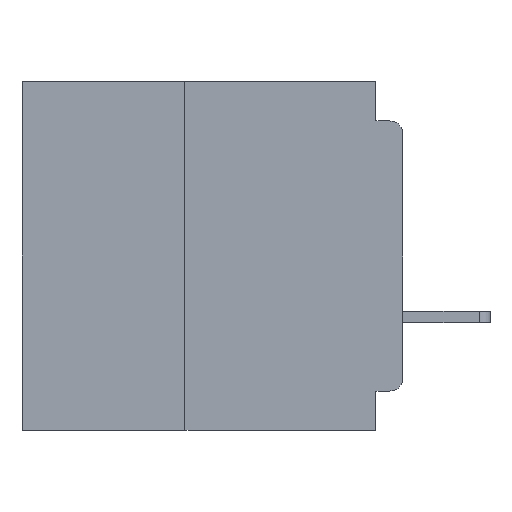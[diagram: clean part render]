
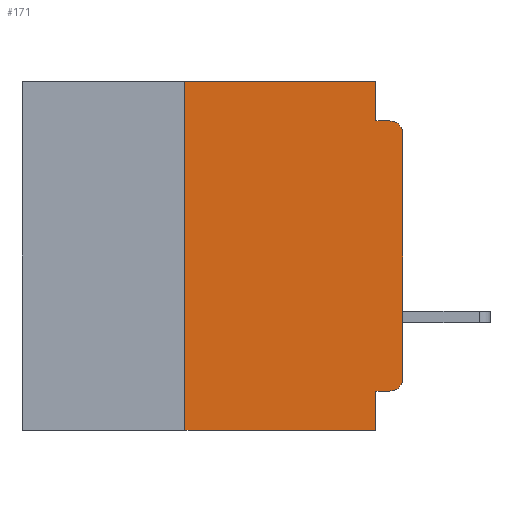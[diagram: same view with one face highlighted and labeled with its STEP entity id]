
A CAD part, left-side view. The second image highlights one B-rep face of the part: STEP entity #171.
In plain terms, the highlighted planar face has unit normal (-1, 0, 0).
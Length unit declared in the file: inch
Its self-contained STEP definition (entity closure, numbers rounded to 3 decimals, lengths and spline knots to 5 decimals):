
#171 = ADVANCED_FACE ( 'NONE', ( #26048 ), #30924, .F. ) ;
#3354 = CARTESIAN_POINT ( 'NONE',  ( 0., 0.031, -0.045 ) ) ;
#3966 = VECTOR ( 'NONE', #53707, 39.37008 ) ;
#3998 = DIRECTION ( 'NONE',  ( 0., 1., 0. ) ) ;
#4062 = DIRECTION ( 'NONE',  ( 1., 0., 0. ) ) ;
#4523 = DIRECTION ( 'NONE',  ( -1., 0., 0. ) ) ;
#5114 = VECTOR ( 'NONE', #3998, 39.37008 ) ;
#5888 = CARTESIAN_POINT ( 'NONE',  ( 0., 0.437, -0.4 ) ) ;
#6887 = EDGE_CURVE ( 'NONE', #55035, #43956, #48521, .T. ) ;
#7261 = ORIENTED_EDGE ( 'NONE', *, *, #20875, .T. ) ;
#7558 = ORIENTED_EDGE ( 'NONE', *, *, #43974, .F. ) ;
#8017 = CIRCLE ( 'NONE', #57983, 0.015 ) ;
#8098 = VERTEX_POINT ( 'NONE', #42284 ) ;
#8631 = ORIENTED_EDGE ( 'NONE', *, *, #9053, .F. ) ;
#8658 = LINE ( 'NONE', #15975, #9285 ) ;
#9053 = EDGE_CURVE ( 'NONE', #44268, #14773, #48695, .T. ) ;
#9285 = VECTOR ( 'NONE', #20602, 39.37008 ) ;
#9909 = DIRECTION ( 'NONE',  ( 0., -1., 0. ) ) ;
#10533 = DIRECTION ( 'NONE',  ( 0., -1., 0. ) ) ;
#10568 = CARTESIAN_POINT ( 'NONE',  ( 0., 0.437, 0. ) ) ;
#10621 = VECTOR ( 'NONE', #9909, 39.37008 ) ;
#11690 = VERTEX_POINT ( 'NONE', #24177 ) ;
#12273 = DIRECTION ( 'NONE',  ( -1., 0., 0. ) ) ;
#12608 = ORIENTED_EDGE ( 'NONE', *, *, #19873, .T. ) ;
#13193 = CARTESIAN_POINT ( 'NONE',  ( 0., 0.031, -0.4 ) ) ;
#13359 = LINE ( 'NONE', #49118, #3966 ) ;
#13393 = AXIS2_PLACEMENT_3D ( 'NONE', #39656, #12273, #44220 ) ;
#13726 = CARTESIAN_POINT ( 'NONE',  ( 0., 0.031, -0.355 ) ) ;
#14773 = VERTEX_POINT ( 'NONE', #58003 ) ;
#15975 = CARTESIAN_POINT ( 'NONE',  ( 0., 0.25, -0.4 ) ) ;
#17292 = LINE ( 'NONE', #35420, #37321 ) ;
#18830 = LINE ( 'NONE', #36121, #5114 ) ;
#18964 = VERTEX_POINT ( 'NONE', #54848 ) ;
#19873 = EDGE_CURVE ( 'NONE', #36688, #11690, #50340, .T. ) ;
#20602 = DIRECTION ( 'NONE',  ( 0., 0., 1. ) ) ;
#20875 = EDGE_CURVE ( 'NONE', #8098, #14773, #30965, .T. ) ;
#21246 = VECTOR ( 'NONE', #46455, 39.37008 ) ;
#22238 = DIRECTION ( 'NONE',  ( 0., 0., -1. ) ) ;
#24177 = CARTESIAN_POINT ( 'NONE',  ( 0., 0., -0.34 ) ) ;
#24867 = EDGE_CURVE ( 'NONE', #11690, #18964, #33382, .T. ) ;
#25678 = AXIS2_PLACEMENT_3D ( 'NONE', #10568, #4062, #46538 ) ;
#26034 = ORIENTED_EDGE ( 'NONE', *, *, #51809, .F. ) ;
#26048 = FACE_OUTER_BOUND ( 'NONE', #56134, .T. ) ;
#29539 = VECTOR ( 'NONE', #10533, 39.37008 ) ;
#30563 = ORIENTED_EDGE ( 'NONE', *, *, #24867, .T. ) ;
#30924 = PLANE ( 'NONE',  #25678 ) ;
#30965 = LINE ( 'NONE', #5888, #29539 ) ;
#32022 = CARTESIAN_POINT ( 'NONE',  ( 0., 0.015, -0.06 ) ) ;
#32921 = CARTESIAN_POINT ( 'NONE',  ( 0., 0., 0. ) ) ;
#33382 = LINE ( 'NONE', #32921, #21246 ) ;
#35420 = CARTESIAN_POINT ( 'NONE',  ( 0., 0.437, 0. ) ) ;
#36121 = CARTESIAN_POINT ( 'NONE',  ( 0., 0., -0.355 ) ) ;
#36631 = DIRECTION ( 'NONE',  ( 0., 0., -1. ) ) ;
#36688 = VERTEX_POINT ( 'NONE', #52552 ) ;
#36721 = CARTESIAN_POINT ( 'NONE',  ( 0., 0.031, 0. ) ) ;
#37321 = VECTOR ( 'NONE', #39970, 39.37008 ) ;
#38124 = ORIENTED_EDGE ( 'NONE', *, *, #41726, .F. ) ;
#39656 = CARTESIAN_POINT ( 'NONE',  ( 0., 0.015, -0.34 ) ) ;
#39970 = DIRECTION ( 'NONE',  ( 0., -1., 0. ) ) ;
#41726 = EDGE_CURVE ( 'NONE', #53040, #44532, #17292, .T. ) ;
#42284 = CARTESIAN_POINT ( 'NONE',  ( 0., 0.25, -0.4 ) ) ;
#43956 = VERTEX_POINT ( 'NONE', #56855 ) ;
#43974 = EDGE_CURVE ( 'NONE', #8098, #53040, #8658, .T. ) ;
#44220 = DIRECTION ( 'NONE',  ( 0., 0., -1. ) ) ;
#44268 = VERTEX_POINT ( 'NONE', #13726 ) ;
#44532 = VERTEX_POINT ( 'NONE', #36721 ) ;
#45748 = ORIENTED_EDGE ( 'NONE', *, *, #6887, .F. ) ;
#45841 = ORIENTED_EDGE ( 'NONE', *, *, #52492, .T. ) ;
#46455 = DIRECTION ( 'NONE',  ( 0., 0., 1. ) ) ;
#46538 = DIRECTION ( 'NONE',  ( 0., 0., -1. ) ) ;
#47413 = CARTESIAN_POINT ( 'NONE',  ( 0., 0.25, 0. ) ) ;
#48521 = LINE ( 'NONE', #55472, #10621 ) ;
#48695 = LINE ( 'NONE', #13193, #57942 ) ;
#49118 = CARTESIAN_POINT ( 'NONE',  ( 0., 0.031, 0. ) ) ;
#50340 = CIRCLE ( 'NONE', #13393, 0.015 ) ;
#51809 = EDGE_CURVE ( 'NONE', #36688, #44268, #18830, .T. ) ;
#52492 = EDGE_CURVE ( 'NONE', #18964, #43956, #8017, .T. ) ;
#52552 = CARTESIAN_POINT ( 'NONE',  ( 0., 0.015, -0.355 ) ) ;
#53040 = VERTEX_POINT ( 'NONE', #47413 ) ;
#53707 = DIRECTION ( 'NONE',  ( 0., 0., -1. ) ) ;
#54848 = CARTESIAN_POINT ( 'NONE',  ( 0., 0., -0.06 ) ) ;
#55035 = VERTEX_POINT ( 'NONE', #3354 ) ;
#55472 = CARTESIAN_POINT ( 'NONE',  ( 0., 0., -0.045 ) ) ;
#55689 = EDGE_CURVE ( 'NONE', #44532, #55035, #13359, .T. ) ;
#56134 = EDGE_LOOP ( 'NONE', ( #30563, #45841, #45748, #56294, #38124, #7558, #7261, #8631, #26034, #12608 ) ) ;
#56294 = ORIENTED_EDGE ( 'NONE', *, *, #55689, .F. ) ;
#56855 = CARTESIAN_POINT ( 'NONE',  ( 0., 0.015, -0.045 ) ) ;
#57942 = VECTOR ( 'NONE', #22238, 39.37008 ) ;
#57983 = AXIS2_PLACEMENT_3D ( 'NONE', #32022, #4523, #36631 ) ;
#58003 = CARTESIAN_POINT ( 'NONE',  ( 0., 0.031, -0.4 ) ) ;
